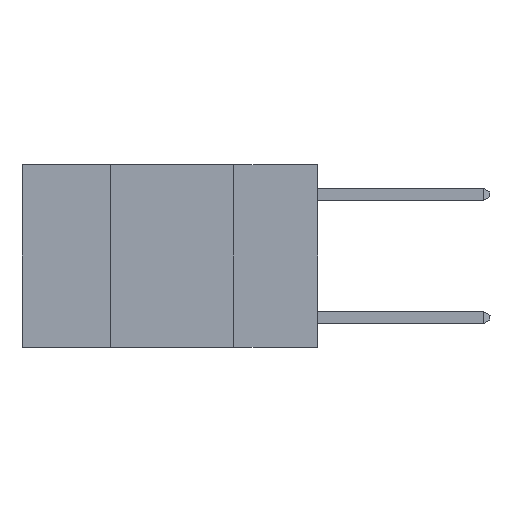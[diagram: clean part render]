
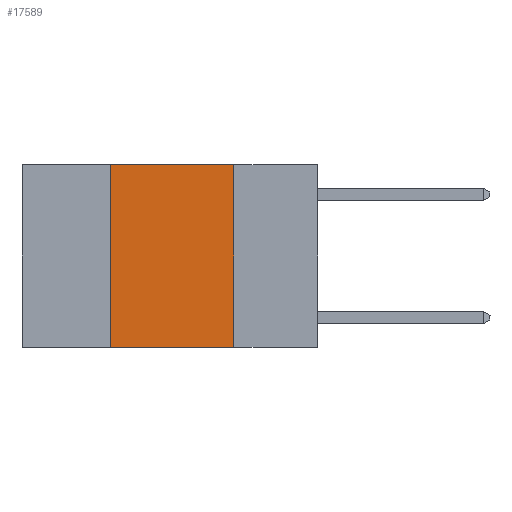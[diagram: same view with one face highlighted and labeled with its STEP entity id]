
A CAD part, left-side view. The second image highlights one B-rep face of the part: STEP entity #17589.
In plain terms, the highlighted planar face has unit normal (-1, 0, 0).
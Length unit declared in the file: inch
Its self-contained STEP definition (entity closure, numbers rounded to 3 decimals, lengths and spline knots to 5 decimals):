
#64 = LINE ( 'NONE', #7256, #11736 ) ;
#375 = EDGE_CURVE ( 'NONE', #17978, #3879, #14467, .T. ) ;
#1196 = EDGE_CURVE ( 'NONE', #17978, #10982, #10506, .T. ) ;
#1464 = EDGE_CURVE ( 'NONE', #5348, #3879, #10952, .T. ) ;
#1576 = ORIENTED_EDGE ( 'NONE', *, *, #375, .T. ) ;
#2043 = EDGE_LOOP ( 'NONE', ( #3436, #4054, #3265, #1576 ) ) ;
#2550 = DIRECTION ( 'NONE',  ( 0., 0., -1. ) ) ;
#3265 = ORIENTED_EDGE ( 'NONE', *, *, #1196, .F. ) ;
#3436 = ORIENTED_EDGE ( 'NONE', *, *, #1464, .F. ) ;
#3879 = VERTEX_POINT ( 'NONE', #9559 ) ;
#4054 = ORIENTED_EDGE ( 'NONE', *, *, #9262, .F. ) ;
#5032 = FACE_OUTER_BOUND ( 'NONE', #2043, .T. ) ;
#5256 = CARTESIAN_POINT ( 'NONE',  ( 0., 0.42, 0. ) ) ;
#5348 = VERTEX_POINT ( 'NONE', #11136 ) ;
#6583 = VECTOR ( 'NONE', #12362, 39.37008 ) ;
#6989 = VECTOR ( 'NONE', #8102, 39.37008 ) ;
#7256 = CARTESIAN_POINT ( 'NONE',  ( 0., 0.6, 0. ) ) ;
#8102 = DIRECTION ( 'NONE',  ( 0., 0., -1. ) ) ;
#8333 = AXIS2_PLACEMENT_3D ( 'NONE', #10003, #11580, #2550 ) ;
#8427 = CARTESIAN_POINT ( 'NONE',  ( 0., 0.17, 0. ) ) ;
#8753 = DIRECTION ( 'NONE',  ( 0., -1., 0. ) ) ;
#9262 = EDGE_CURVE ( 'NONE', #10982, #5348, #64, .T. ) ;
#9559 = CARTESIAN_POINT ( 'NONE',  ( 0., 0.17, -0.37 ) ) ;
#10003 = CARTESIAN_POINT ( 'NONE',  ( 0., 0.6, 0. ) ) ;
#10506 = LINE ( 'NONE', #14270, #13962 ) ;
#10952 = LINE ( 'NONE', #8427, #6989 ) ;
#10982 = VERTEX_POINT ( 'NONE', #5256 ) ;
#11136 = CARTESIAN_POINT ( 'NONE',  ( 0., 0.17, 0. ) ) ;
#11580 = DIRECTION ( 'NONE',  ( 1., 0., 0. ) ) ;
#11736 = VECTOR ( 'NONE', #8753, 39.37008 ) ;
#12264 = CARTESIAN_POINT ( 'NONE',  ( 0., 0.6, -0.37 ) ) ;
#12362 = DIRECTION ( 'NONE',  ( 0., -1., 0. ) ) ;
#13962 = VECTOR ( 'NONE', #14357, 39.37008 ) ;
#14270 = CARTESIAN_POINT ( 'NONE',  ( 0., 0.42, 0. ) ) ;
#14357 = DIRECTION ( 'NONE',  ( 0., 0., 1. ) ) ;
#14467 = LINE ( 'NONE', #12264, #6583 ) ;
#15271 = CARTESIAN_POINT ( 'NONE',  ( 0., 0.42, -0.37 ) ) ;
#17347 = PLANE ( 'NONE',  #8333 ) ;
#17589 = ADVANCED_FACE ( 'NONE', ( #5032 ), #17347, .F. ) ;
#17978 = VERTEX_POINT ( 'NONE', #15271 ) ;
